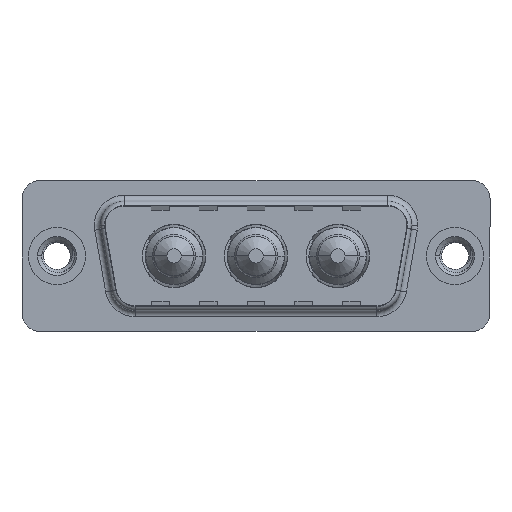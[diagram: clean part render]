
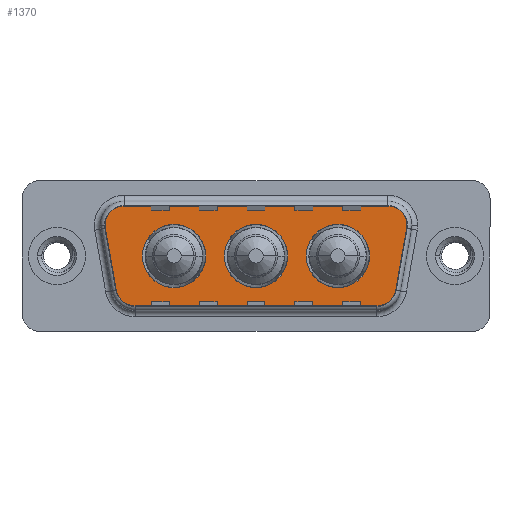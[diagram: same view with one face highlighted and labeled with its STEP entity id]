
A CAD part, top view. The second image highlights one B-rep face of the part: STEP entity #1370.
In plain terms, the highlighted planar face has unit normal (0, 0, 1).
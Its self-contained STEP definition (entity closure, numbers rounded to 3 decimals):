
#33 = EDGE_CURVE ( 'NONE', #12377, #9196, #8833, .T. ) ;
#111 = AXIS2_PLACEMENT_3D ( 'NONE', #3855, #9619, #4625 ) ;
#173 = EDGE_CURVE ( 'NONE', #5126, #2486, #7894, .T. ) ;
#308 = DIRECTION ( 'NONE',  ( 1., 0., 0. ) ) ;
#315 = ORIENTED_EDGE ( 'NONE', *, *, #4115, .F. ) ;
#397 = FACE_BOUND ( 'NONE', #9582, .T. ) ;
#605 = CARTESIAN_POINT ( 'NONE',  ( 29.889, 2.9, 0. ) ) ;
#889 = EDGE_CURVE ( 'NONE', #4946, #10469, #6009, .T. ) ;
#1039 = CARTESIAN_POINT ( 'NONE',  ( 3.441, 2.553, 0. ) ) ;
#1326 = ORIENTED_EDGE ( 'NONE', *, *, #8400, .T. ) ;
#1351 = AXIS2_PLACEMENT_3D ( 'NONE', #4853, #5139, #5088 ) ;
#1370 = ADVANCED_FACE ( 'NONE', ( #397, #3035, #10764, #8069 ), #7936, .T. ) ;
#1410 = CARTESIAN_POINT ( 'NONE',  ( 29.859, 2.553, 0. ) ) ;
#1524 = DIRECTION ( 'NONE',  ( 1., 0., 0. ) ) ;
#1547 = DIRECTION ( 'NONE',  ( 0., 0., 1. ) ) ;
#1616 = CARTESIAN_POINT ( 'NONE',  ( 16.65, 0., 0. ) ) ;
#2195 = CIRCLE ( 'NONE', #12518, 2. ) ;
#2306 = EDGE_CURVE ( 'NONE', #9196, #12377, #7580, .T. ) ;
#2389 = DIRECTION ( 'NONE',  ( 0., 0., 1. ) ) ;
#2422 = DIRECTION ( 'NONE',  ( 1., 0., 0. ) ) ;
#2486 = VERTEX_POINT ( 'NONE', #5597 ) ;
#2505 = LINE ( 'NONE', #9527, #5820 ) ;
#2567 = VECTOR ( 'NONE', #4213, 1000. ) ;
#2634 = EDGE_CURVE ( 'NONE', #9553, #5718, #11542, .T. ) ;
#2639 = AXIS2_PLACEMENT_3D ( 'NONE', #11477, #2389, #308 ) ;
#2710 = CARTESIAN_POINT ( 'NONE',  ( 4.464, -3.247, 0. ) ) ;
#2859 = CIRCLE ( 'NONE', #5112, 2. ) ;
#2878 = DIRECTION ( 'NONE',  ( 0., 0., 1. ) ) ;
#2896 = VERTEX_POINT ( 'NONE', #2710 ) ;
#2910 = AXIS2_PLACEMENT_3D ( 'NONE', #1616, #1547, #1524 ) ;
#3035 = FACE_BOUND ( 'NONE', #9991, .T. ) ;
#3062 = DIRECTION ( 'NONE',  ( -1., 0., 0. ) ) ;
#3079 = CARTESIAN_POINT ( 'NONE',  ( 14., 0., 0. ) ) ;
#3117 = DIRECTION ( 'NONE',  ( 0., 0., 1. ) ) ;
#3141 = DIRECTION ( 'NONE',  ( 0., 0., 1. ) ) ;
#3422 = ORIENTED_EDGE ( 'NONE', *, *, #9493, .T. ) ;
#3594 = EDGE_CURVE ( 'NONE', #11049, #12381, #10708, .T. ) ;
#3734 = CARTESIAN_POINT ( 'NONE',  ( 28.836, -3.247, 0. ) ) ;
#3763 = DIRECTION ( 'NONE',  ( 0.174, -0.985, 0. ) ) ;
#3807 = ORIENTED_EDGE ( 'NONE', *, *, #5503, .T. ) ;
#3855 = CARTESIAN_POINT ( 'NONE',  ( 27.889, 2.9, 0. ) ) ;
#3986 = ORIENTED_EDGE ( 'NONE', *, *, #6056, .T. ) ;
#4078 = CARTESIAN_POINT ( 'NONE',  ( 19.3, 0., 0. ) ) ;
#4100 = LINE ( 'NONE', #6026, #11524 ) ;
#4115 = EDGE_CURVE ( 'NONE', #10469, #4946, #11525, .T. ) ;
#4213 = DIRECTION ( 'NONE',  ( 0.174, 0.985, 0. ) ) ;
#4342 = DIRECTION ( 'NONE',  ( 0., 0., 1. ) ) ;
#4613 = CARTESIAN_POINT ( 'NONE',  ( 6.434, -2.9, 0. ) ) ;
#4625 = DIRECTION ( 'NONE',  ( -1., 0., 0. ) ) ;
#4756 = EDGE_CURVE ( 'NONE', #12334, #2896, #2505, .T. ) ;
#4853 = CARTESIAN_POINT ( 'NONE',  ( 9.8, 0., 0. ) ) ;
#4946 = VERTEX_POINT ( 'NONE', #6165 ) ;
#5088 = DIRECTION ( 'NONE',  ( 1., 0., 0. ) ) ;
#5095 = ORIENTED_EDGE ( 'NONE', *, *, #4756, .T. ) ;
#5112 = AXIS2_PLACEMENT_3D ( 'NONE', #11997, #5942, #13013 ) ;
#5126 = VERTEX_POINT ( 'NONE', #605 ) ;
#5139 = DIRECTION ( 'NONE',  ( 0., 0., 1. ) ) ;
#5503 = EDGE_CURVE ( 'NONE', #8369, #5126, #9647, .T. ) ;
#5597 = CARTESIAN_POINT ( 'NONE',  ( 27.889, 4.9, 0. ) ) ;
#5630 = DIRECTION ( 'NONE',  ( -1., 0., 0. ) ) ;
#5718 = VERTEX_POINT ( 'NONE', #9066 ) ;
#5820 = VECTOR ( 'NONE', #3763, 1000. ) ;
#5841 = ORIENTED_EDGE ( 'NONE', *, *, #173, .T. ) ;
#5942 = DIRECTION ( 'NONE',  ( 0., 0., 1. ) ) ;
#6009 = CIRCLE ( 'NONE', #7660, 2.65 ) ;
#6026 = CARTESIAN_POINT ( 'NONE',  ( 5.411, 4.9, 0. ) ) ;
#6056 = EDGE_CURVE ( 'NONE', #6754, #8369, #7900, .T. ) ;
#6067 = DIRECTION ( 'NONE',  ( 1., 0., 0. ) ) ;
#6079 = CARTESIAN_POINT ( 'NONE',  ( 26.866, -2.9, 0. ) ) ;
#6165 = CARTESIAN_POINT ( 'NONE',  ( 12.45, 0., 0. ) ) ;
#6291 = DIRECTION ( 'NONE',  ( 0., 0., 1. ) ) ;
#6368 = EDGE_CURVE ( 'NONE', #5718, #6754, #9455, .T. ) ;
#6455 = DIRECTION ( 'NONE',  ( 0., 0., 1. ) ) ;
#6740 = CARTESIAN_POINT ( 'NONE',  ( 20.85, 0., 0. ) ) ;
#6754 = VERTEX_POINT ( 'NONE', #3734 ) ;
#7304 = CARTESIAN_POINT ( 'NONE',  ( 6.434, -4.9, 0. ) ) ;
#7340 = CARTESIAN_POINT ( 'NONE',  ( 26.866, -2.9, 0. ) ) ;
#7545 = CARTESIAN_POINT ( 'NONE',  ( 29.859, 2.553, 0. ) ) ;
#7580 = CIRCLE ( 'NONE', #2639, 2.65 ) ;
#7617 = CARTESIAN_POINT ( 'NONE',  ( 23.5, 0., 0. ) ) ;
#7660 = AXIS2_PLACEMENT_3D ( 'NONE', #10935, #2878, #10955 ) ;
#7894 = CIRCLE ( 'NONE', #111, 2. ) ;
#7900 = LINE ( 'NONE', #1410, #2567 ) ;
#7936 = PLANE ( 'NONE',  #8482 ) ;
#8068 = ORIENTED_EDGE ( 'NONE', *, *, #6368, .T. ) ;
#8069 = FACE_OUTER_BOUND ( 'NONE', #9734, .T. ) ;
#8369 = VERTEX_POINT ( 'NONE', #7545 ) ;
#8400 = EDGE_CURVE ( 'NONE', #2896, #9553, #2195, .T. ) ;
#8404 = AXIS2_PLACEMENT_3D ( 'NONE', #7617, #6291, #9240 ) ;
#8482 = AXIS2_PLACEMENT_3D ( 'NONE', #7340, #6455, #6067 ) ;
#8703 = ORIENTED_EDGE ( 'NONE', *, *, #11015, .T. ) ;
#8804 = VECTOR ( 'NONE', #2422, 1000. ) ;
#8833 = CIRCLE ( 'NONE', #8404, 2.65 ) ;
#8861 = ORIENTED_EDGE ( 'NONE', *, *, #2306, .F. ) ;
#9038 = CARTESIAN_POINT ( 'NONE',  ( 6.434, -4.9, 0. ) ) ;
#9066 = CARTESIAN_POINT ( 'NONE',  ( 26.866, -4.9, 0. ) ) ;
#9088 = CARTESIAN_POINT ( 'NONE',  ( 26.15, 0., 0. ) ) ;
#9137 = CARTESIAN_POINT ( 'NONE',  ( 16.65, 0., 0. ) ) ;
#9196 = VERTEX_POINT ( 'NONE', #6740 ) ;
#9208 = ORIENTED_EDGE ( 'NONE', *, *, #2634, .T. ) ;
#9240 = DIRECTION ( 'NONE',  ( 1., 0., 0. ) ) ;
#9455 = CIRCLE ( 'NONE', #11372, 2. ) ;
#9493 = EDGE_CURVE ( 'NONE', #9788, #12334, #2859, .T. ) ;
#9527 = CARTESIAN_POINT ( 'NONE',  ( 3.441, 2.553, 0. ) ) ;
#9553 = VERTEX_POINT ( 'NONE', #9038 ) ;
#9582 = EDGE_LOOP ( 'NONE', ( #9989, #10806 ) ) ;
#9619 = DIRECTION ( 'NONE',  ( 0., 0., 1. ) ) ;
#9647 = CIRCLE ( 'NONE', #10185, 2. ) ;
#9734 = EDGE_LOOP ( 'NONE', ( #8068, #3986, #3807, #5841, #8703, #3422, #5095, #1326, #9208 ) ) ;
#9788 = VERTEX_POINT ( 'NONE', #12355 ) ;
#9989 = ORIENTED_EDGE ( 'NONE', *, *, #3594, .F. ) ;
#9991 = EDGE_LOOP ( 'NONE', ( #10002, #8861 ) ) ;
#10002 = ORIENTED_EDGE ( 'NONE', *, *, #33, .F. ) ;
#10169 = DIRECTION ( 'NONE',  ( 1., 0., 0. ) ) ;
#10185 = AXIS2_PLACEMENT_3D ( 'NONE', #10856, #3141, #3062 ) ;
#10297 = CARTESIAN_POINT ( 'NONE',  ( 7.15, 0., 0. ) ) ;
#10361 = DIRECTION ( 'NONE',  ( 1., 0., 0. ) ) ;
#10469 = VERTEX_POINT ( 'NONE', #10297 ) ;
#10708 = CIRCLE ( 'NONE', #2910, 2.65 ) ;
#10764 = FACE_BOUND ( 'NONE', #11515, .T. ) ;
#10806 = ORIENTED_EDGE ( 'NONE', *, *, #12389, .F. ) ;
#10856 = CARTESIAN_POINT ( 'NONE',  ( 27.889, 2.9, 0. ) ) ;
#10935 = CARTESIAN_POINT ( 'NONE',  ( 9.8, 0., 0. ) ) ;
#10955 = DIRECTION ( 'NONE',  ( 1., 0., 0. ) ) ;
#11015 = EDGE_CURVE ( 'NONE', #2486, #9788, #4100, .T. ) ;
#11049 = VERTEX_POINT ( 'NONE', #4078 ) ;
#11372 = AXIS2_PLACEMENT_3D ( 'NONE', #6079, #4342, #10361 ) ;
#11477 = CARTESIAN_POINT ( 'NONE',  ( 23.5, 0., 0. ) ) ;
#11515 = EDGE_LOOP ( 'NONE', ( #11609, #315 ) ) ;
#11524 = VECTOR ( 'NONE', #12097, 1000. ) ;
#11525 = CIRCLE ( 'NONE', #1351, 2.65 ) ;
#11542 = LINE ( 'NONE', #7304, #8804 ) ;
#11609 = ORIENTED_EDGE ( 'NONE', *, *, #889, .F. ) ;
#11686 = DIRECTION ( 'NONE',  ( 0., 0., 1. ) ) ;
#11841 = CIRCLE ( 'NONE', #12075, 2.65 ) ;
#11997 = CARTESIAN_POINT ( 'NONE',  ( 5.411, 2.9, 0. ) ) ;
#12075 = AXIS2_PLACEMENT_3D ( 'NONE', #9137, #3117, #10169 ) ;
#12097 = DIRECTION ( 'NONE',  ( -1., 0., 0. ) ) ;
#12334 = VERTEX_POINT ( 'NONE', #1039 ) ;
#12355 = CARTESIAN_POINT ( 'NONE',  ( 5.411, 4.9, 0. ) ) ;
#12377 = VERTEX_POINT ( 'NONE', #9088 ) ;
#12381 = VERTEX_POINT ( 'NONE', #3079 ) ;
#12389 = EDGE_CURVE ( 'NONE', #12381, #11049, #11841, .T. ) ;
#12518 = AXIS2_PLACEMENT_3D ( 'NONE', #4613, #11686, #5630 ) ;
#13013 = DIRECTION ( 'NONE',  ( 1., 0., 0. ) ) ;
